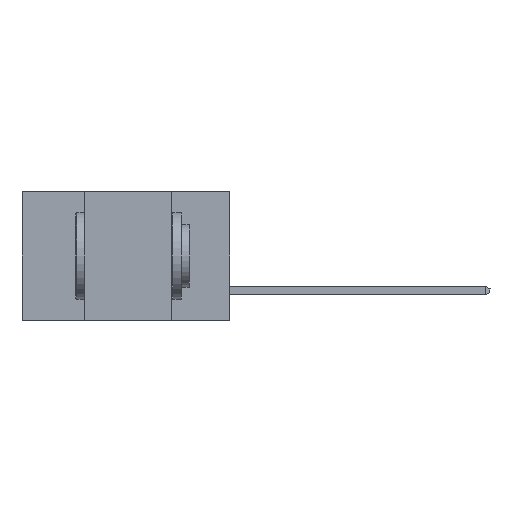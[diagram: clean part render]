
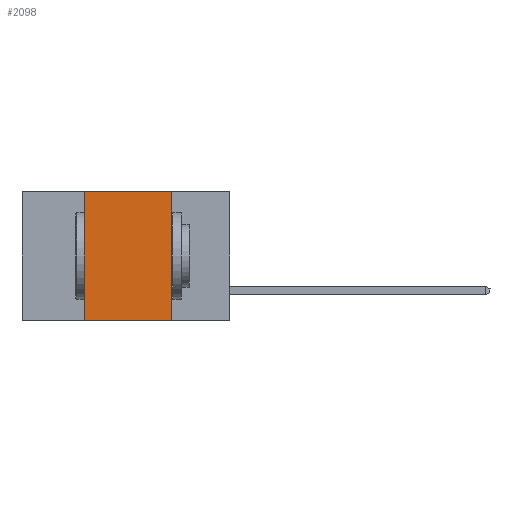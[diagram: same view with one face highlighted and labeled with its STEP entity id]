
A CAD part, left-side view. The second image highlights one B-rep face of the part: STEP entity #2098.
In plain terms, the highlighted planar face has unit normal (-1, 0, 0).
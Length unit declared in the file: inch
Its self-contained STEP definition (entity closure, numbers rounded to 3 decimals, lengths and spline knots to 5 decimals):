
#1314 = LINE ( 'NONE', #2964, #12460 ) ;
#1863 = LINE ( 'NONE', #12409, #7065 ) ;
#1900 = CARTESIAN_POINT ( 'NONE',  ( 0., 0.42, -0.37 ) ) ;
#2098 = ADVANCED_FACE ( 'NONE', ( #8209 ), #6724, .F. ) ;
#2336 = CARTESIAN_POINT ( 'NONE',  ( 0., 0.17, 0. ) ) ;
#2964 = CARTESIAN_POINT ( 'NONE',  ( 0., 0.17, -0.37 ) ) ;
#3898 = VERTEX_POINT ( 'NONE', #2336 ) ;
#4343 = ORIENTED_EDGE ( 'NONE', *, *, #13267, .F. ) ;
#4538 = VERTEX_POINT ( 'NONE', #7870 ) ;
#4856 = CARTESIAN_POINT ( 'NONE',  ( 0., 0.42, 0. ) ) ;
#5220 = ORIENTED_EDGE ( 'NONE', *, *, #7278, .T. ) ;
#6724 = PLANE ( 'NONE',  #12514 ) ;
#6776 = ORIENTED_EDGE ( 'NONE', *, *, #14601, .F. ) ;
#7065 = VECTOR ( 'NONE', #7815, 39.37008 ) ;
#7278 = EDGE_CURVE ( 'NONE', #8381, #4538, #1863, .T. ) ;
#7581 = CARTESIAN_POINT ( 'NONE',  ( 0., 0.6, 0. ) ) ;
#7815 = DIRECTION ( 'NONE',  ( 0., -1., 0. ) ) ;
#7870 = CARTESIAN_POINT ( 'NONE',  ( 0., 0.17, -0.37 ) ) ;
#8209 = FACE_OUTER_BOUND ( 'NONE', #9441, .T. ) ;
#8381 = VERTEX_POINT ( 'NONE', #11964 ) ;
#9441 = EDGE_LOOP ( 'NONE', ( #16246, #6776, #4343, #5220 ) ) ;
#9872 = DIRECTION ( 'NONE',  ( 0., 0., -1. ) ) ;
#10436 = DIRECTION ( 'NONE',  ( 0., -1., 0. ) ) ;
#11343 = DIRECTION ( 'NONE',  ( 1., 0., 0. ) ) ;
#11964 = CARTESIAN_POINT ( 'NONE',  ( 0., 0.42, -0.37 ) ) ;
#12409 = CARTESIAN_POINT ( 'NONE',  ( 0., 0.6, -0.37 ) ) ;
#12460 = VECTOR ( 'NONE', #14771, 39.37008 ) ;
#12514 = AXIS2_PLACEMENT_3D ( 'NONE', #12702, #11343, #9872 ) ;
#12702 = CARTESIAN_POINT ( 'NONE',  ( 0., 0.6, 0. ) ) ;
#13267 = EDGE_CURVE ( 'NONE', #8381, #15925, #13613, .T. ) ;
#13596 = EDGE_CURVE ( 'NONE', #3898, #4538, #1314, .T. ) ;
#13613 = LINE ( 'NONE', #1900, #13740 ) ;
#13740 = VECTOR ( 'NONE', #15172, 39.37008 ) ;
#14601 = EDGE_CURVE ( 'NONE', #15925, #3898, #16449, .T. ) ;
#14771 = DIRECTION ( 'NONE',  ( 0., 0., -1. ) ) ;
#15172 = DIRECTION ( 'NONE',  ( 0., 0., 1. ) ) ;
#15925 = VERTEX_POINT ( 'NONE', #4856 ) ;
#16246 = ORIENTED_EDGE ( 'NONE', *, *, #13596, .F. ) ;
#16449 = LINE ( 'NONE', #7581, #18708 ) ;
#18708 = VECTOR ( 'NONE', #10436, 39.37008 ) ;
